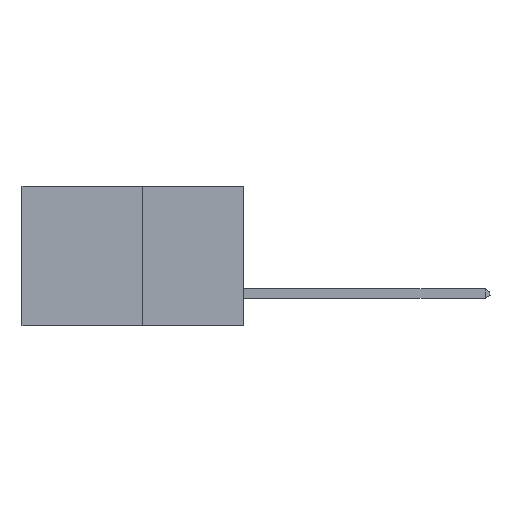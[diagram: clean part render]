
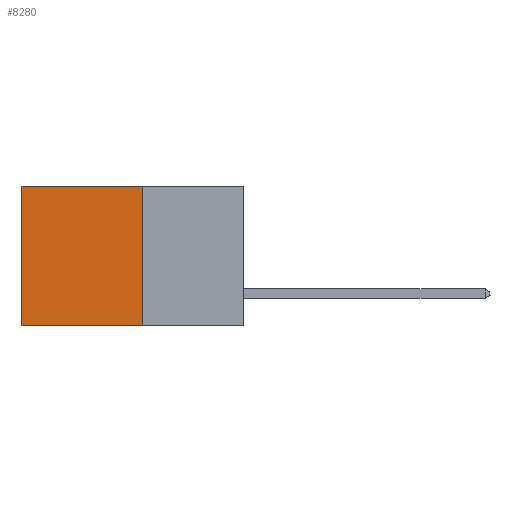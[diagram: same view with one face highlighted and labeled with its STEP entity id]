
A CAD part, left-side view. The second image highlights one B-rep face of the part: STEP entity #8280.
In plain terms, the highlighted planar face has unit normal (-1, 0, 0).
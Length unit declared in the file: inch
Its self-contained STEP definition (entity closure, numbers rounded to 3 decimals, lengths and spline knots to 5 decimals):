
#197 = DIRECTION ( 'NONE',  ( 0., 1., 0. ) ) ;
#288 = CARTESIAN_POINT ( 'NONE',  ( 0.277, 0.27, 0. ) ) ;
#320 = EDGE_LOOP ( 'NONE', ( #9956, #497, #1187, #2208 ) ) ;
#497 = ORIENTED_EDGE ( 'NONE', *, *, #2696, .F. ) ;
#1187 = ORIENTED_EDGE ( 'NONE', *, *, #8804, .F. ) ;
#2152 = VERTEX_POINT ( 'NONE', #9396 ) ;
#2208 = ORIENTED_EDGE ( 'NONE', *, *, #5486, .T. ) ;
#2627 = LINE ( 'NONE', #5647, #4513 ) ;
#2691 = CARTESIAN_POINT ( 'NONE',  ( 0.277, 0.27, -0.37 ) ) ;
#2696 = EDGE_CURVE ( 'NONE', #9272, #11311, #8647, .T. ) ;
#2827 = CARTESIAN_POINT ( 'NONE',  ( 0.277, 0.59, -0.37 ) ) ;
#2829 = DIRECTION ( 'NONE',  ( 0., 0., -1. ) ) ;
#3616 = LINE ( 'NONE', #2827, #12061 ) ;
#4429 = LINE ( 'NONE', #288, #10300 ) ;
#4483 = EDGE_CURVE ( 'NONE', #5001, #11311, #3616, .T. ) ;
#4494 = CARTESIAN_POINT ( 'NONE',  ( 0.277, 0.59, -0.37 ) ) ;
#4513 = VECTOR ( 'NONE', #12263, 39.37008 ) ;
#4893 = PLANE ( 'NONE',  #13045 ) ;
#5001 = VERTEX_POINT ( 'NONE', #7786 ) ;
#5346 = DIRECTION ( 'NONE',  ( 0., 1., 0. ) ) ;
#5486 = EDGE_CURVE ( 'NONE', #2152, #5001, #4429, .T. ) ;
#5647 = CARTESIAN_POINT ( 'NONE',  ( 0.277, 0.27, -0.37 ) ) ;
#5770 = VECTOR ( 'NONE', #5346, 39.37008 ) ;
#5969 = DIRECTION ( 'NONE',  ( 0., 0., -1. ) ) ;
#7401 = CARTESIAN_POINT ( 'NONE',  ( 0.277, 0.27, -0.37 ) ) ;
#7718 = FACE_OUTER_BOUND ( 'NONE', #320, .T. ) ;
#7786 = CARTESIAN_POINT ( 'NONE',  ( 0.277, 0.59, 0. ) ) ;
#8280 = ADVANCED_FACE ( 'NONE', ( #7718 ), #4893, .F. ) ;
#8647 = LINE ( 'NONE', #8844, #5770 ) ;
#8804 = EDGE_CURVE ( 'NONE', #2152, #9272, #2627, .T. ) ;
#8844 = CARTESIAN_POINT ( 'NONE',  ( 0.277, 0.27, -0.37 ) ) ;
#9272 = VERTEX_POINT ( 'NONE', #7401 ) ;
#9396 = CARTESIAN_POINT ( 'NONE',  ( 0.277, 0.27, 0. ) ) ;
#9956 = ORIENTED_EDGE ( 'NONE', *, *, #4483, .T. ) ;
#10300 = VECTOR ( 'NONE', #197, 39.37008 ) ;
#11311 = VERTEX_POINT ( 'NONE', #4494 ) ;
#12061 = VECTOR ( 'NONE', #2829, 39.37008 ) ;
#12263 = DIRECTION ( 'NONE',  ( 0., 0., -1. ) ) ;
#12600 = DIRECTION ( 'NONE',  ( 1., 0., 0. ) ) ;
#13045 = AXIS2_PLACEMENT_3D ( 'NONE', #2691, #12600, #5969 ) ;
